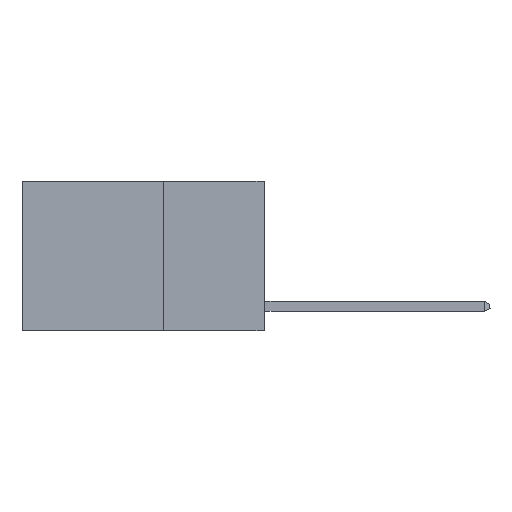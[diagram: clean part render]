
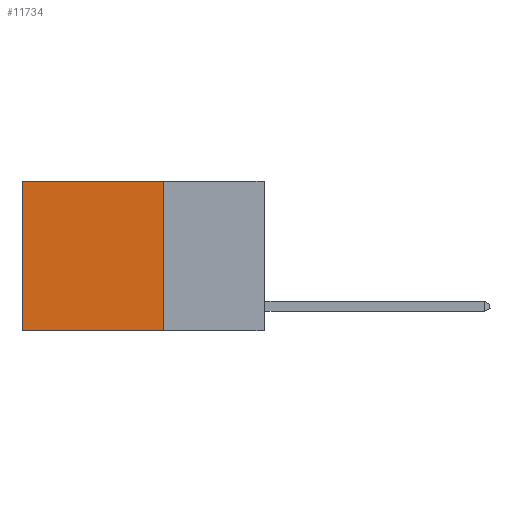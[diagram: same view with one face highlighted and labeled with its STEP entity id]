
A CAD part, left-side view. The second image highlights one B-rep face of the part: STEP entity #11734.
In plain terms, the highlighted planar face has unit normal (-1, 0, 0).
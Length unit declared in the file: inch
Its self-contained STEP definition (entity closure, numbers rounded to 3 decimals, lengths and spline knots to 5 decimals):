
#237 = FACE_OUTER_BOUND ( 'NONE', #405, .T. ) ;
#405 = EDGE_LOOP ( 'NONE', ( #5612, #3920, #4199, #8239 ) ) ;
#427 = EDGE_CURVE ( 'NONE', #18077, #13211, #4261, .T. ) ;
#1718 = EDGE_CURVE ( 'NONE', #18077, #2539, #3852, .T. ) ;
#2065 = DIRECTION ( 'NONE',  ( 0., 0., -1. ) ) ;
#2539 = VERTEX_POINT ( 'NONE', #19650 ) ;
#3043 = CARTESIAN_POINT ( 'NONE',  ( 0.2625, 0.6, 0. ) ) ;
#3375 = DIRECTION ( 'NONE',  ( 0., 0., -1. ) ) ;
#3431 = DIRECTION ( 'NONE',  ( 0., 1., 0. ) ) ;
#3852 = LINE ( 'NONE', #3954, #13817 ) ;
#3920 = ORIENTED_EDGE ( 'NONE', *, *, #19403, .F. ) ;
#3954 = CARTESIAN_POINT ( 'NONE',  ( 0.2625, 0.25, 0. ) ) ;
#4199 = ORIENTED_EDGE ( 'NONE', *, *, #1718, .F. ) ;
#4261 = LINE ( 'NONE', #14660, #17129 ) ;
#4265 = DIRECTION ( 'NONE',  ( 0., 0., -1. ) ) ;
#5612 = ORIENTED_EDGE ( 'NONE', *, *, #5721, .T. ) ;
#5721 = EDGE_CURVE ( 'NONE', #13211, #10163, #13230, .T. ) ;
#6899 = CARTESIAN_POINT ( 'NONE',  ( 0.2625, 0.25, 0. ) ) ;
#7311 = AXIS2_PLACEMENT_3D ( 'NONE', #6899, #17103, #2065 ) ;
#8100 = DIRECTION ( 'NONE',  ( 0., 1., 0. ) ) ;
#8239 = ORIENTED_EDGE ( 'NONE', *, *, #427, .T. ) ;
#9253 = VECTOR ( 'NONE', #3431, 39.37008 ) ;
#10163 = VERTEX_POINT ( 'NONE', #15170 ) ;
#10546 = LINE ( 'NONE', #17254, #9253 ) ;
#11734 = ADVANCED_FACE ( 'NONE', ( #237 ), #20153, .F. ) ;
#13211 = VERTEX_POINT ( 'NONE', #3043 ) ;
#13230 = LINE ( 'NONE', #18299, #13884 ) ;
#13817 = VECTOR ( 'NONE', #4265, 39.37008 ) ;
#13884 = VECTOR ( 'NONE', #3375, 39.37008 ) ;
#14660 = CARTESIAN_POINT ( 'NONE',  ( 0.2625, 0.25, 0. ) ) ;
#15170 = CARTESIAN_POINT ( 'NONE',  ( 0.2625, 0.6, -0.37 ) ) ;
#17103 = DIRECTION ( 'NONE',  ( 1., 0., 0. ) ) ;
#17129 = VECTOR ( 'NONE', #8100, 39.37008 ) ;
#17254 = CARTESIAN_POINT ( 'NONE',  ( 0.2625, 0.25, -0.37 ) ) ;
#18077 = VERTEX_POINT ( 'NONE', #20383 ) ;
#18299 = CARTESIAN_POINT ( 'NONE',  ( 0.2625, 0.6, 0. ) ) ;
#19403 = EDGE_CURVE ( 'NONE', #2539, #10163, #10546, .T. ) ;
#19650 = CARTESIAN_POINT ( 'NONE',  ( 0.2625, 0.25, -0.37 ) ) ;
#20153 = PLANE ( 'NONE',  #7311 ) ;
#20383 = CARTESIAN_POINT ( 'NONE',  ( 0.2625, 0.25, 0. ) ) ;
